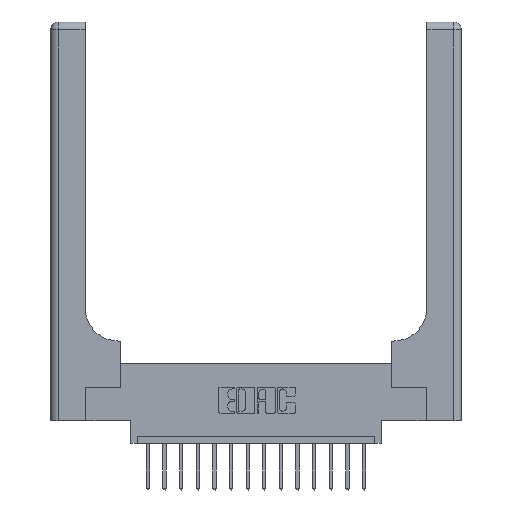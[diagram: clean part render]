
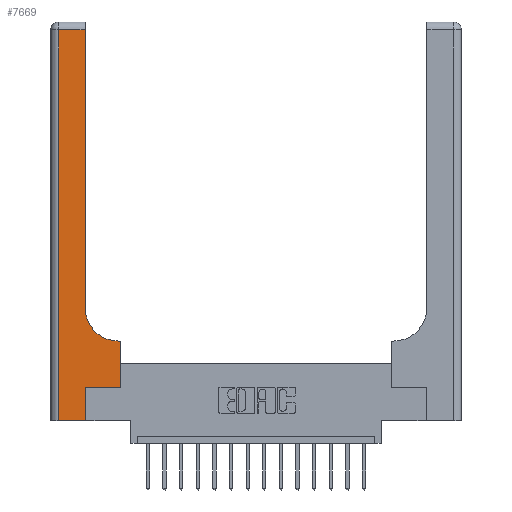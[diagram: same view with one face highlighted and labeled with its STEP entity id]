
A CAD part, top view. The second image highlights one B-rep face of the part: STEP entity #7669.
In plain terms, the highlighted planar face has unit normal (0, 0, 1).
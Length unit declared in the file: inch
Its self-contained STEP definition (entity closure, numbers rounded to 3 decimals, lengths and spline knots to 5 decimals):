
#184 = DIRECTION ( 'NONE',  ( 0., 1., 0. ) ) ;
#262 = PLANE ( 'NONE',  #16996 ) ;
#264 = CARTESIAN_POINT ( 'NONE',  ( 0.265, 0.25, 0.37 ) ) ;
#519 = DIRECTION ( 'NONE',  ( -1., 0., 0. ) ) ;
#565 = CARTESIAN_POINT ( 'NONE',  ( 0.06, 2.94, 0.37 ) ) ;
#640 = CARTESIAN_POINT ( 'NONE',  ( 0.265, 0., 0.37 ) ) ;
#1291 = VERTEX_POINT ( 'NONE', #8043 ) ;
#1360 = CARTESIAN_POINT ( 'NONE',  ( 0.528, 0.6, 0.37 ) ) ;
#1486 = VERTEX_POINT ( 'NONE', #1360 ) ;
#1727 = CARTESIAN_POINT ( 'NONE',  ( 0.265, 0., 0.37 ) ) ;
#1753 = DIRECTION ( 'NONE',  ( 0., 0., -1. ) ) ;
#1779 = EDGE_CURVE ( 'NONE', #1291, #14381, #5670, .T. ) ;
#2530 = DIRECTION ( 'NONE',  ( 0., -1., 0. ) ) ;
#2820 = CARTESIAN_POINT ( 'NONE',  ( 0.51, 0.6, 0.37 ) ) ;
#3065 = EDGE_CURVE ( 'NONE', #15263, #1291, #15735, .T. ) ;
#3156 = DIRECTION ( 'NONE',  ( -1., 0., 0. ) ) ;
#3435 = VECTOR ( 'NONE', #15983, 39.37008 ) ;
#3654 = DIRECTION ( 'NONE',  ( 0., 1., 0. ) ) ;
#3787 = ORIENTED_EDGE ( 'NONE', *, *, #17154, .T. ) ;
#4241 = CARTESIAN_POINT ( 'NONE',  ( 0.26, 0.85, 0.37 ) ) ;
#4252 = ORIENTED_EDGE ( 'NONE', *, *, #8919, .T. ) ;
#4529 = EDGE_CURVE ( 'NONE', #5232, #1486, #8416, .T. ) ;
#4623 = CARTESIAN_POINT ( 'NONE',  ( 0.26, 0.6, 0.37 ) ) ;
#4733 = LINE ( 'NONE', #264, #16343 ) ;
#5186 = VERTEX_POINT ( 'NONE', #2820 ) ;
#5232 = VERTEX_POINT ( 'NONE', #7346 ) ;
#5452 = EDGE_CURVE ( 'NONE', #17787, #5232, #4733, .T. ) ;
#5670 = LINE ( 'NONE', #10124, #10250 ) ;
#5765 = ORIENTED_EDGE ( 'NONE', *, *, #3065, .T. ) ;
#5928 = CIRCLE ( 'NONE', #16234, 0.25 ) ;
#5955 = DIRECTION ( 'NONE',  ( 1., 0., 0. ) ) ;
#6029 = EDGE_CURVE ( 'NONE', #6401, #17520, #9038, .T. ) ;
#6217 = VECTOR ( 'NONE', #5955, 39.37008 ) ;
#6354 = DIRECTION ( 'NONE',  ( 1., 0., 0. ) ) ;
#6394 = CARTESIAN_POINT ( 'NONE',  ( 0.528, 0.25, 0.37 ) ) ;
#6401 = VERTEX_POINT ( 'NONE', #6609 ) ;
#6609 = CARTESIAN_POINT ( 'NONE',  ( 0.06, 0., 0.37 ) ) ;
#7346 = CARTESIAN_POINT ( 'NONE',  ( 0.528, 0.25, 0.37 ) ) ;
#7669 = ADVANCED_FACE ( 'NONE', ( #10928 ), #262, .F. ) ;
#7792 = ORIENTED_EDGE ( 'NONE', *, *, #17383, .T. ) ;
#8043 = CARTESIAN_POINT ( 'NONE',  ( 0.26, 2.94, 0.37 ) ) ;
#8102 = VECTOR ( 'NONE', #184, 39.37008 ) ;
#8416 = LINE ( 'NONE', #6394, #3435 ) ;
#8865 = LINE ( 'NONE', #4623, #11835 ) ;
#8919 = EDGE_CURVE ( 'NONE', #1486, #5186, #8865, .T. ) ;
#8965 = CARTESIAN_POINT ( 'NONE',  ( 0.26, 3., 0.37 ) ) ;
#9038 = LINE ( 'NONE', #10098, #6217 ) ;
#10065 = CARTESIAN_POINT ( 'NONE',  ( 0., 3., 0.37 ) ) ;
#10098 = CARTESIAN_POINT ( 'NONE',  ( 0., 0., 0.37 ) ) ;
#10124 = CARTESIAN_POINT ( 'NONE',  ( 0., 2.94, 0.37 ) ) ;
#10250 = VECTOR ( 'NONE', #16977, 39.37008 ) ;
#10301 = VECTOR ( 'NONE', #2530, 39.37008 ) ;
#10516 = ORIENTED_EDGE ( 'NONE', *, *, #12670, .T. ) ;
#10827 = CARTESIAN_POINT ( 'NONE',  ( 0.06, 3., 0.37 ) ) ;
#10928 = FACE_OUTER_BOUND ( 'NONE', #16766, .T. ) ;
#11023 = ORIENTED_EDGE ( 'NONE', *, *, #6029, .T. ) ;
#11835 = VECTOR ( 'NONE', #519, 39.37008 ) ;
#12092 = VECTOR ( 'NONE', #3654, 39.37008 ) ;
#12476 = ORIENTED_EDGE ( 'NONE', *, *, #4529, .T. ) ;
#12670 = EDGE_CURVE ( 'NONE', #5186, #15263, #5928, .T. ) ;
#14381 = VERTEX_POINT ( 'NONE', #565 ) ;
#14753 = LINE ( 'NONE', #10827, #10301 ) ;
#15263 = VERTEX_POINT ( 'NONE', #4241 ) ;
#15735 = LINE ( 'NONE', #8965, #12092 ) ;
#15857 = DIRECTION ( 'NONE',  ( 0., 0., -1. ) ) ;
#15983 = DIRECTION ( 'NONE',  ( 0., 1., 0. ) ) ;
#16234 = AXIS2_PLACEMENT_3D ( 'NONE', #17249, #15857, #17304 ) ;
#16281 = CARTESIAN_POINT ( 'NONE',  ( 0.265, 0.25, 0.37 ) ) ;
#16343 = VECTOR ( 'NONE', #6354, 39.37008 ) ;
#16664 = ORIENTED_EDGE ( 'NONE', *, *, #5452, .T. ) ;
#16766 = EDGE_LOOP ( 'NONE', ( #5765, #16930, #3787, #11023, #7792, #16664, #12476, #4252, #10516 ) ) ;
#16889 = LINE ( 'NONE', #1727, #8102 ) ;
#16930 = ORIENTED_EDGE ( 'NONE', *, *, #1779, .T. ) ;
#16977 = DIRECTION ( 'NONE',  ( -1., 0., 0. ) ) ;
#16996 = AXIS2_PLACEMENT_3D ( 'NONE', #10065, #1753, #3156 ) ;
#17154 = EDGE_CURVE ( 'NONE', #14381, #6401, #14753, .T. ) ;
#17249 = CARTESIAN_POINT ( 'NONE',  ( 0.51, 0.85, 0.37 ) ) ;
#17304 = DIRECTION ( 'NONE',  ( 1., 0., 0. ) ) ;
#17383 = EDGE_CURVE ( 'NONE', #17520, #17787, #16889, .T. ) ;
#17520 = VERTEX_POINT ( 'NONE', #640 ) ;
#17787 = VERTEX_POINT ( 'NONE', #16281 ) ;
